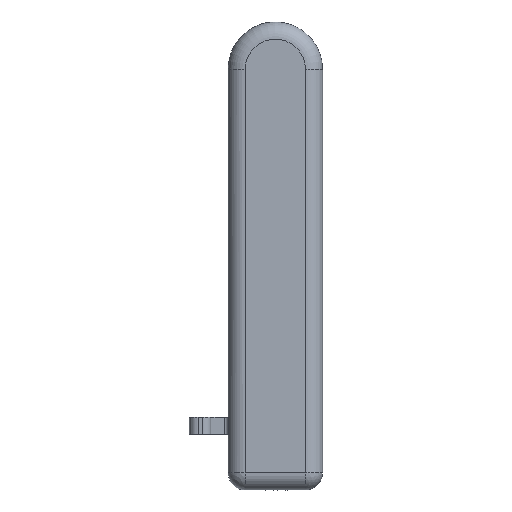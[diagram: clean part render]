
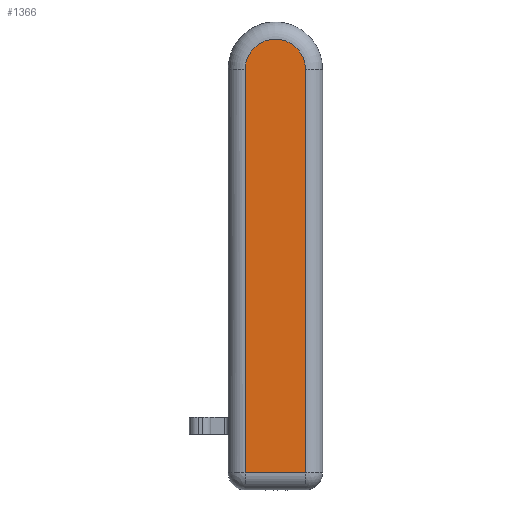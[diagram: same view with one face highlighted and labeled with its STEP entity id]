
A CAD part, front view. The second image highlights one B-rep face of the part: STEP entity #1366.
In plain terms, the highlighted planar face has unit normal (0, -1, 0).
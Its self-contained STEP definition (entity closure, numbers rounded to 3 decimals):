
#921=CARTESIAN_POINT('',(7.,-11.0,5.0));
#922=VERTEX_POINT('',#921);
#954=CARTESIAN_POINT('',(7.,-11.0,99.0));
#955=VERTEX_POINT('',#954);
#963=CARTESIAN_POINT('',(7.,-11.0,99.0));
#964=DIRECTION('',(0.0,0.0,-1.0));
#965=VECTOR('',#964,94.0);
#966=LINE('',#963,#965);
#967=EDGE_CURVE('',#955,#922,#966,.T.);
#1035=CARTESIAN_POINT('',(-7.,-11.0,5.0));
#1036=VERTEX_POINT('',#1035);
#1141=CARTESIAN_POINT('',(-7.,-11.0,99.0));
#1142=VERTEX_POINT('',#1141);
#1143=CARTESIAN_POINT('',(-7.,-11.0,5.0));
#1144=DIRECTION('',(0.0,0.0,1.0));
#1145=VECTOR('',#1144,94.);
#1146=LINE('',#1143,#1145);
#1147=EDGE_CURVE('',#1036,#1142,#1146,.T.);
#1176=CARTESIAN_POINT('',(0.,-11.0,99.0));
#1177=DIRECTION('',(0.0,1.0,0.0));
#1178=DIRECTION('',(0.0,0.0,1.0));
#1179=AXIS2_PLACEMENT_3D('',#1176,#1177,#1178);
#1180=CIRCLE('',#1179,7.);
#1181=EDGE_CURVE('',#1142,#955,#1180,.T.);
#1192=CARTESIAN_POINT('',(7.,-11.0,5.0));
#1193=DIRECTION('',(-1.0,0.0,0.0));
#1194=VECTOR('',#1193,14.);
#1195=LINE('',#1192,#1194);
#1196=EDGE_CURVE('',#922,#1036,#1195,.T.);
#1355=CARTESIAN_POINT('',(0.,-11.0,99.));
#1356=DIRECTION('',(0.0,1.0,0.0));
#1357=DIRECTION('',(0.0,0.0,1.0));
#1358=AXIS2_PLACEMENT_3D('',#1355,#1356,#1357);
#1359=PLANE('',#1358);
#1360=ORIENTED_EDGE('',*,*,#1147,.F.);
#1361=ORIENTED_EDGE('',*,*,#1196,.F.);
#1362=ORIENTED_EDGE('',*,*,#967,.F.);
#1363=ORIENTED_EDGE('',*,*,#1181,.F.);
#1364=EDGE_LOOP('',(#1360,#1361,#1362,#1363));
#1365=FACE_OUTER_BOUND('',#1364,.T.);
#1366=ADVANCED_FACE('',(#1365),#1359,.F.);
